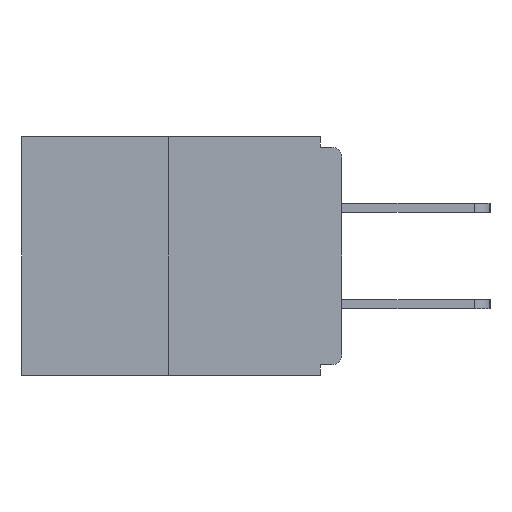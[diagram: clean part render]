
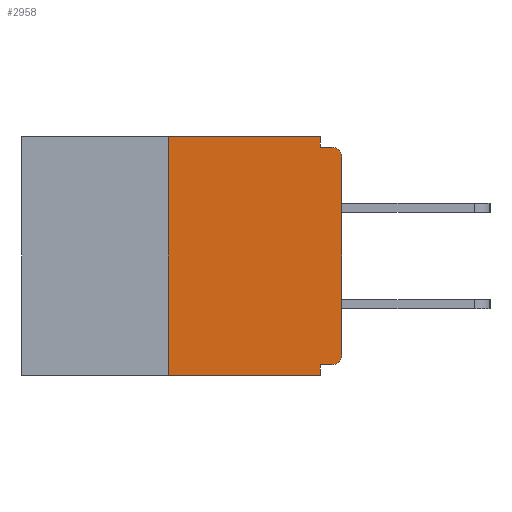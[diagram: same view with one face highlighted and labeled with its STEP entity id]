
A CAD part, left-side view. The second image highlights one B-rep face of the part: STEP entity #2958.
In plain terms, the highlighted planar face has unit normal (-1, 0, 0).
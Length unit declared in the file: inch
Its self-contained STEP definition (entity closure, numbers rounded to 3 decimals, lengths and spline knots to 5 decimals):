
#156 = AXIS2_PLACEMENT_3D ( 'NONE', #12147, #13141, #3494 ) ;
#405 = DIRECTION ( 'NONE',  ( -1., 0., 0. ) ) ;
#640 = LINE ( 'NONE', #9229, #6360 ) ;
#1108 = VERTEX_POINT ( 'NONE', #12600 ) ;
#1300 = CARTESIAN_POINT ( 'NONE',  ( 0., 0.031, -0.343 ) ) ;
#1569 = VERTEX_POINT ( 'NONE', #6855 ) ;
#1573 = CARTESIAN_POINT ( 'NONE',  ( 0., 0., -0.328 ) ) ;
#1803 = CIRCLE ( 'NONE', #8606, 0.015 ) ;
#1919 = CARTESIAN_POINT ( 'NONE',  ( 0., 0., -0.313 ) ) ;
#2032 = CIRCLE ( 'NONE', #9986, 0.015 ) ;
#2320 = VERTEX_POINT ( 'NONE', #2471 ) ;
#2449 = EDGE_CURVE ( 'NONE', #13992, #3507, #2032, .T. ) ;
#2471 = CARTESIAN_POINT ( 'NONE',  ( 0., 0.015, -0.328 ) ) ;
#2637 = DIRECTION ( 'NONE',  ( 0., 1., 0. ) ) ;
#2780 = LINE ( 'NONE', #1573, #10082 ) ;
#2803 = VERTEX_POINT ( 'NONE', #9560 ) ;
#2958 = ADVANCED_FACE ( 'NONE', ( #8770 ), #9981, .F. ) ;
#2997 = CARTESIAN_POINT ( 'NONE',  ( 0., 0.015, -0.03 ) ) ;
#3054 = ORIENTED_EDGE ( 'NONE', *, *, #3791, .T. ) ;
#3184 = LINE ( 'NONE', #7446, #13010 ) ;
#3196 = ORIENTED_EDGE ( 'NONE', *, *, #5504, .F. ) ;
#3494 = DIRECTION ( 'NONE',  ( 0., 0., -1. ) ) ;
#3507 = VERTEX_POINT ( 'NONE', #12968 ) ;
#3579 = VECTOR ( 'NONE', #7939, 39.37008 ) ;
#3660 = VECTOR ( 'NONE', #9979, 39.37008 ) ;
#3718 = LINE ( 'NONE', #12019, #4557 ) ;
#3757 = VERTEX_POINT ( 'NONE', #5538 ) ;
#3791 = EDGE_CURVE ( 'NONE', #11667, #13992, #13662, .T. ) ;
#3925 = ORIENTED_EDGE ( 'NONE', *, *, #9227, .T. ) ;
#4127 = DIRECTION ( 'NONE',  ( -1., 0., 0. ) ) ;
#4557 = VECTOR ( 'NONE', #5932, 39.37008 ) ;
#4592 = EDGE_CURVE ( 'NONE', #3757, #11349, #7262, .T. ) ;
#4665 = CARTESIAN_POINT ( 'NONE',  ( 0., 0., 0. ) ) ;
#5018 = EDGE_CURVE ( 'NONE', #2803, #3507, #10323, .T. ) ;
#5504 = EDGE_CURVE ( 'NONE', #1569, #1108, #640, .T. ) ;
#5538 = CARTESIAN_POINT ( 'NONE',  ( 0., 0.25, -0.343 ) ) ;
#5932 = DIRECTION ( 'NONE',  ( 0., 0., -1. ) ) ;
#6205 = DIRECTION ( 'NONE',  ( 0., -1., 0. ) ) ;
#6360 = VECTOR ( 'NONE', #11231, 39.37008 ) ;
#6482 = DIRECTION ( 'NONE',  ( 0., 0., -1. ) ) ;
#6855 = CARTESIAN_POINT ( 'NONE',  ( 0., 0.25, 0. ) ) ;
#6968 = LINE ( 'NONE', #1300, #3660 ) ;
#7262 = LINE ( 'NONE', #9410, #9425 ) ;
#7424 = EDGE_LOOP ( 'NONE', ( #3196, #11238, #8803, #13016, #9082, #3925, #3054, #9363, #9326, #8623 ) ) ;
#7446 = CARTESIAN_POINT ( 'NONE',  ( 0., 0.25, 0. ) ) ;
#7694 = EDGE_CURVE ( 'NONE', #1108, #2803, #3718, .T. ) ;
#7939 = DIRECTION ( 'NONE',  ( 0., 0., 1. ) ) ;
#7989 = EDGE_CURVE ( 'NONE', #12903, #11349, #6968, .T. ) ;
#8606 = AXIS2_PLACEMENT_3D ( 'NONE', #9057, #405, #8921 ) ;
#8623 = ORIENTED_EDGE ( 'NONE', *, *, #7694, .F. ) ;
#8770 = FACE_OUTER_BOUND ( 'NONE', #7424, .T. ) ;
#8803 = ORIENTED_EDGE ( 'NONE', *, *, #4592, .T. ) ;
#8921 = DIRECTION ( 'NONE',  ( 0., 0., -1. ) ) ;
#9057 = CARTESIAN_POINT ( 'NONE',  ( 0., 0.015, -0.313 ) ) ;
#9082 = ORIENTED_EDGE ( 'NONE', *, *, #13855, .F. ) ;
#9107 = DIRECTION ( 'NONE',  ( 0., -1., 0. ) ) ;
#9177 = CARTESIAN_POINT ( 'NONE',  ( 0., 0., -0.015 ) ) ;
#9227 = EDGE_CURVE ( 'NONE', #2320, #11667, #1803, .T. ) ;
#9229 = CARTESIAN_POINT ( 'NONE',  ( 0., 0.46, 0. ) ) ;
#9326 = ORIENTED_EDGE ( 'NONE', *, *, #5018, .F. ) ;
#9363 = ORIENTED_EDGE ( 'NONE', *, *, #2449, .T. ) ;
#9410 = CARTESIAN_POINT ( 'NONE',  ( 0., 0.46, -0.343 ) ) ;
#9425 = VECTOR ( 'NONE', #6205, 39.37008 ) ;
#9560 = CARTESIAN_POINT ( 'NONE',  ( 0., 0.031, -0.015 ) ) ;
#9613 = CARTESIAN_POINT ( 'NONE',  ( 0., 0., -0.03 ) ) ;
#9740 = DIRECTION ( 'NONE',  ( 0., 0., 1. ) ) ;
#9979 = DIRECTION ( 'NONE',  ( 0., 0., -1. ) ) ;
#9981 = PLANE ( 'NONE',  #156 ) ;
#9986 = AXIS2_PLACEMENT_3D ( 'NONE', #2997, #4127, #6482 ) ;
#10082 = VECTOR ( 'NONE', #2637, 39.37008 ) ;
#10323 = LINE ( 'NONE', #9177, #13886 ) ;
#11231 = DIRECTION ( 'NONE',  ( 0., -1., 0. ) ) ;
#11238 = ORIENTED_EDGE ( 'NONE', *, *, #11613, .F. ) ;
#11349 = VERTEX_POINT ( 'NONE', #13337 ) ;
#11613 = EDGE_CURVE ( 'NONE', #3757, #1569, #3184, .T. ) ;
#11667 = VERTEX_POINT ( 'NONE', #1919 ) ;
#12019 = CARTESIAN_POINT ( 'NONE',  ( 0., 0.031, 0. ) ) ;
#12038 = CARTESIAN_POINT ( 'NONE',  ( 0., 0.031, -0.328 ) ) ;
#12147 = CARTESIAN_POINT ( 'NONE',  ( 0., 0.46, 0. ) ) ;
#12600 = CARTESIAN_POINT ( 'NONE',  ( 0., 0.031, 0. ) ) ;
#12903 = VERTEX_POINT ( 'NONE', #12038 ) ;
#12968 = CARTESIAN_POINT ( 'NONE',  ( 0., 0.015, -0.015 ) ) ;
#13010 = VECTOR ( 'NONE', #9740, 39.37008 ) ;
#13016 = ORIENTED_EDGE ( 'NONE', *, *, #7989, .F. ) ;
#13141 = DIRECTION ( 'NONE',  ( 1., 0., 0. ) ) ;
#13337 = CARTESIAN_POINT ( 'NONE',  ( 0., 0.031, -0.343 ) ) ;
#13662 = LINE ( 'NONE', #4665, #3579 ) ;
#13855 = EDGE_CURVE ( 'NONE', #2320, #12903, #2780, .T. ) ;
#13886 = VECTOR ( 'NONE', #9107, 39.37008 ) ;
#13992 = VERTEX_POINT ( 'NONE', #9613 ) ;
